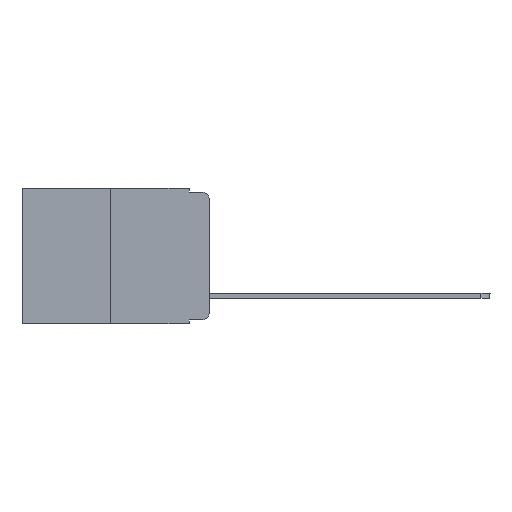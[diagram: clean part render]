
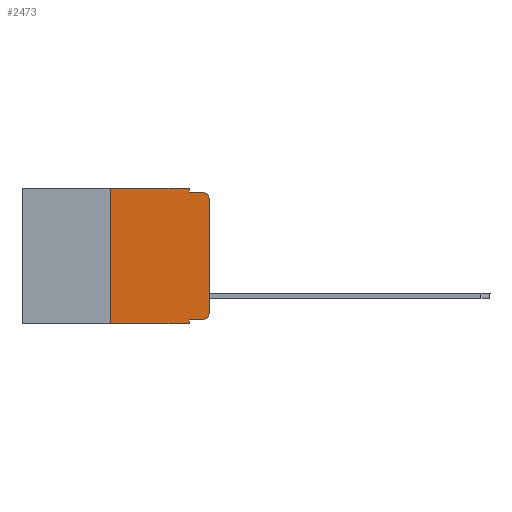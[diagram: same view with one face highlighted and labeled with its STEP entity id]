
A CAD part, left-side view. The second image highlights one B-rep face of the part: STEP entity #2473.
In plain terms, the highlighted planar face has unit normal (-1, 0, 0).
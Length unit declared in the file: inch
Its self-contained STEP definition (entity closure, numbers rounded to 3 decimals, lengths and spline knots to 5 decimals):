
#128 = LINE ( 'NONE', #16274, #4537 ) ;
#395 = VECTOR ( 'NONE', #8750, 39.37008 ) ;
#625 = CARTESIAN_POINT ( 'NONE',  ( 0., 0.051, 0. ) ) ;
#1019 = EDGE_CURVE ( 'NONE', #15595, #13791, #16594, .T. ) ;
#1091 = CIRCLE ( 'NONE', #15697, 0.02 ) ;
#1410 = LINE ( 'NONE', #18831, #13814 ) ;
#1567 = DIRECTION ( 'NONE',  ( -1., 0., 0. ) ) ;
#2172 = EDGE_CURVE ( 'NONE', #19134, #15595, #128, .T. ) ;
#2473 = ADVANCED_FACE ( 'NONE', ( #2546 ), #18895, .F. ) ;
#2546 = FACE_OUTER_BOUND ( 'NONE', #8587, .T. ) ;
#2585 = CARTESIAN_POINT ( 'NONE',  ( 0., 0.02, -0.333 ) ) ;
#2741 = EDGE_CURVE ( 'NONE', #5995, #4770, #13606, .T. ) ;
#2916 = VECTOR ( 'NONE', #19859, 39.37008 ) ;
#3260 = EDGE_CURVE ( 'NONE', #5469, #19134, #1410, .T. ) ;
#3289 = CARTESIAN_POINT ( 'NONE',  ( 0., 0.25, 0. ) ) ;
#3425 = LINE ( 'NONE', #6403, #20131 ) ;
#3576 = EDGE_CURVE ( 'NONE', #13791, #13925, #3932, .T. ) ;
#3893 = VERTEX_POINT ( 'NONE', #16054 ) ;
#3932 = LINE ( 'NONE', #20098, #4283 ) ;
#4105 = VECTOR ( 'NONE', #10464, 39.37008 ) ;
#4283 = VECTOR ( 'NONE', #8755, 39.37008 ) ;
#4500 = CARTESIAN_POINT ( 'NONE',  ( 0., 0.02, -0.03 ) ) ;
#4537 = VECTOR ( 'NONE', #4889, 39.37008 ) ;
#4735 = CARTESIAN_POINT ( 'NONE',  ( 0., 0.02, -0.313 ) ) ;
#4770 = VERTEX_POINT ( 'NONE', #14047 ) ;
#4889 = DIRECTION ( 'NONE',  ( 0., -1., 0. ) ) ;
#5469 = VERTEX_POINT ( 'NONE', #12047 ) ;
#5995 = VERTEX_POINT ( 'NONE', #14146 ) ;
#6126 = EDGE_CURVE ( 'NONE', #3893, #17426, #17637, .T. ) ;
#6178 = ORIENTED_EDGE ( 'NONE', *, *, #16477, .T. ) ;
#6197 = ORIENTED_EDGE ( 'NONE', *, *, #3260, .F. ) ;
#6274 = CARTESIAN_POINT ( 'NONE',  ( 0., 0., 0. ) ) ;
#6403 = CARTESIAN_POINT ( 'NONE',  ( 0., 0.473, -0.343 ) ) ;
#6573 = EDGE_CURVE ( 'NONE', #11612, #3893, #19632, .T. ) ;
#6803 = ORIENTED_EDGE ( 'NONE', *, *, #2172, .F. ) ;
#7901 = DIRECTION ( 'NONE',  ( 0., 0., 1. ) ) ;
#8587 = EDGE_LOOP ( 'NONE', ( #13434, #6178, #18520, #10840, #6803, #6197, #18559, #20453, #13477, #14932 ) ) ;
#8750 = DIRECTION ( 'NONE',  ( 0., 0., -1. ) ) ;
#8755 = DIRECTION ( 'NONE',  ( 0., -1., 0. ) ) ;
#10464 = DIRECTION ( 'NONE',  ( 0., -1., 0. ) ) ;
#10840 = ORIENTED_EDGE ( 'NONE', *, *, #1019, .F. ) ;
#11006 = DIRECTION ( 'NONE',  ( -1., 0., 0. ) ) ;
#11317 = AXIS2_PLACEMENT_3D ( 'NONE', #14138, #17119, #17213 ) ;
#11612 = VERTEX_POINT ( 'NONE', #2585 ) ;
#11697 = CARTESIAN_POINT ( 'NONE',  ( 0., 0.02, -0.01 ) ) ;
#11821 = AXIS2_PLACEMENT_3D ( 'NONE', #4735, #1567, #12954 ) ;
#11941 = CARTESIAN_POINT ( 'NONE',  ( 0., 0.051, -0.333 ) ) ;
#12047 = CARTESIAN_POINT ( 'NONE',  ( 0., 0.25, -0.343 ) ) ;
#12954 = DIRECTION ( 'NONE',  ( 0., 0., -1. ) ) ;
#13434 = ORIENTED_EDGE ( 'NONE', *, *, #6126, .T. ) ;
#13477 = ORIENTED_EDGE ( 'NONE', *, *, #15322, .T. ) ;
#13550 = LINE ( 'NONE', #11941, #4105 ) ;
#13606 = LINE ( 'NONE', #625, #2916 ) ;
#13791 = VERTEX_POINT ( 'NONE', #17768 ) ;
#13814 = VECTOR ( 'NONE', #7901, 39.37008 ) ;
#13925 = VERTEX_POINT ( 'NONE', #11697 ) ;
#14047 = CARTESIAN_POINT ( 'NONE',  ( 0., 0.051, -0.343 ) ) ;
#14138 = CARTESIAN_POINT ( 'NONE',  ( 0., 0.473, 0. ) ) ;
#14146 = CARTESIAN_POINT ( 'NONE',  ( 0., 0.051, -0.333 ) ) ;
#14389 = CARTESIAN_POINT ( 'NONE',  ( 0., 0.051, 0. ) ) ;
#14400 = CARTESIAN_POINT ( 'NONE',  ( 0., 0., -0.03 ) ) ;
#14597 = DIRECTION ( 'NONE',  ( 0., -1., 0. ) ) ;
#14932 = ORIENTED_EDGE ( 'NONE', *, *, #6573, .T. ) ;
#15220 = CARTESIAN_POINT ( 'NONE',  ( 0., 0.051, 0. ) ) ;
#15322 = EDGE_CURVE ( 'NONE', #5995, #11612, #13550, .T. ) ;
#15595 = VERTEX_POINT ( 'NONE', #14389 ) ;
#15697 = AXIS2_PLACEMENT_3D ( 'NONE', #4500, #11006, #17488 ) ;
#16054 = CARTESIAN_POINT ( 'NONE',  ( 0., 0., -0.313 ) ) ;
#16274 = CARTESIAN_POINT ( 'NONE',  ( 0., 0.473, 0. ) ) ;
#16477 = EDGE_CURVE ( 'NONE', #17426, #13925, #1091, .T. ) ;
#16594 = LINE ( 'NONE', #15220, #395 ) ;
#17119 = DIRECTION ( 'NONE',  ( 1., 0., 0. ) ) ;
#17213 = DIRECTION ( 'NONE',  ( 0., 0., -1. ) ) ;
#17426 = VERTEX_POINT ( 'NONE', #14400 ) ;
#17473 = EDGE_CURVE ( 'NONE', #5469, #4770, #3425, .T. ) ;
#17488 = DIRECTION ( 'NONE',  ( 0., 0., -1. ) ) ;
#17637 = LINE ( 'NONE', #6274, #20291 ) ;
#17768 = CARTESIAN_POINT ( 'NONE',  ( 0., 0.051, -0.01 ) ) ;
#18520 = ORIENTED_EDGE ( 'NONE', *, *, #3576, .F. ) ;
#18559 = ORIENTED_EDGE ( 'NONE', *, *, #17473, .T. ) ;
#18831 = CARTESIAN_POINT ( 'NONE',  ( 0., 0.25, 0. ) ) ;
#18895 = PLANE ( 'NONE',  #11317 ) ;
#19134 = VERTEX_POINT ( 'NONE', #3289 ) ;
#19542 = DIRECTION ( 'NONE',  ( 0., 0., 1. ) ) ;
#19632 = CIRCLE ( 'NONE', #11821, 0.02 ) ;
#19859 = DIRECTION ( 'NONE',  ( 0., 0., -1. ) ) ;
#20098 = CARTESIAN_POINT ( 'NONE',  ( 0., 0.051, -0.01 ) ) ;
#20131 = VECTOR ( 'NONE', #14597, 39.37008 ) ;
#20291 = VECTOR ( 'NONE', #19542, 39.37008 ) ;
#20453 = ORIENTED_EDGE ( 'NONE', *, *, #2741, .F. ) ;
